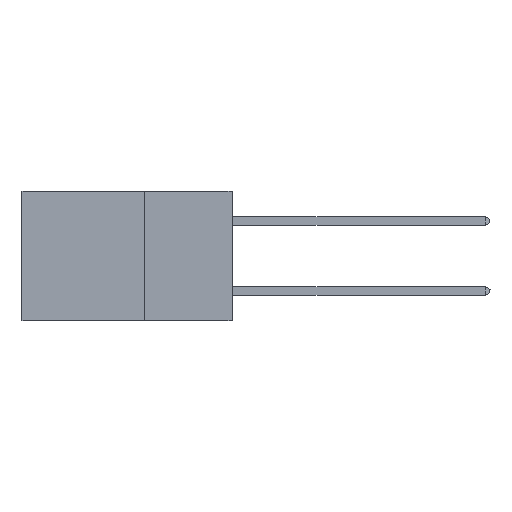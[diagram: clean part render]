
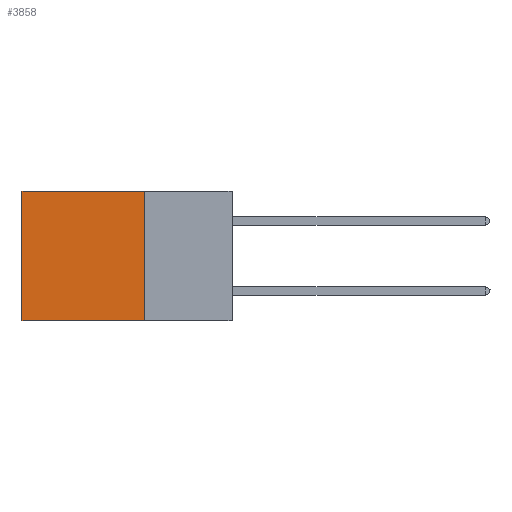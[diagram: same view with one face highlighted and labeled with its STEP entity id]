
A CAD part, left-side view. The second image highlights one B-rep face of the part: STEP entity #3858.
In plain terms, the highlighted planar face has unit normal (-1, 0, 0).
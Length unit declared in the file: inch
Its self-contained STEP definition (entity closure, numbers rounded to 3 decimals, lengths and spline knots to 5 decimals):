
#981 = ORIENTED_EDGE ( 'NONE', *, *, #20808, .T. ) ;
#1035 = DIRECTION ( 'NONE',  ( 0., 0., -1. ) ) ;
#1607 = ORIENTED_EDGE ( 'NONE', *, *, #6414, .T. ) ;
#1695 = DIRECTION ( 'NONE',  ( 0., 1., 0. ) ) ;
#2354 = VERTEX_POINT ( 'NONE', #20238 ) ;
#2769 = FACE_OUTER_BOUND ( 'NONE', #6070, .T. ) ;
#3026 = LINE ( 'NONE', #21168, #22658 ) ;
#3858 = ADVANCED_FACE ( 'NONE', ( #2769 ), #4705, .F. ) ;
#4690 = LINE ( 'NONE', #19210, #17046 ) ;
#4705 = PLANE ( 'NONE',  #22194 ) ;
#4819 = DIRECTION ( 'NONE',  ( 0., 1., 0. ) ) ;
#6070 = EDGE_LOOP ( 'NONE', ( #981, #16297, #16019, #1607 ) ) ;
#6388 = CARTESIAN_POINT ( 'NONE',  ( 0.2875, 0.25, -0.37 ) ) ;
#6414 = EDGE_CURVE ( 'NONE', #7320, #2354, #19826, .T. ) ;
#6417 = CARTESIAN_POINT ( 'NONE',  ( 0.2875, 0.25, 0. ) ) ;
#6467 = DIRECTION ( 'NONE',  ( 0., 0., -1. ) ) ;
#7256 = CARTESIAN_POINT ( 'NONE',  ( 0.2875, 0.25, 0. ) ) ;
#7320 = VERTEX_POINT ( 'NONE', #16934 ) ;
#9088 = VECTOR ( 'NONE', #4819, 39.37008 ) ;
#9526 = DIRECTION ( 'NONE',  ( 0., 0., -1. ) ) ;
#10051 = DIRECTION ( 'NONE',  ( 1., 0., 0. ) ) ;
#12334 = CARTESIAN_POINT ( 'NONE',  ( 0.2875, 0.6, -0.37 ) ) ;
#12747 = LINE ( 'NONE', #7256, #13029 ) ;
#13029 = VECTOR ( 'NONE', #9526, 39.37008 ) ;
#14997 = EDGE_CURVE ( 'NONE', #7320, #18546, #12747, .T. ) ;
#15842 = VERTEX_POINT ( 'NONE', #12334 ) ;
#16019 = ORIENTED_EDGE ( 'NONE', *, *, #14997, .F. ) ;
#16297 = ORIENTED_EDGE ( 'NONE', *, *, #23192, .F. ) ;
#16934 = CARTESIAN_POINT ( 'NONE',  ( 0.2875, 0.25, 0. ) ) ;
#17046 = VECTOR ( 'NONE', #6467, 39.37008 ) ;
#18546 = VERTEX_POINT ( 'NONE', #6388 ) ;
#19210 = CARTESIAN_POINT ( 'NONE',  ( 0.2875, 0.6, 0. ) ) ;
#19826 = LINE ( 'NONE', #22862, #9088 ) ;
#20238 = CARTESIAN_POINT ( 'NONE',  ( 0.2875, 0.6, 0. ) ) ;
#20808 = EDGE_CURVE ( 'NONE', #2354, #15842, #4690, .T. ) ;
#21168 = CARTESIAN_POINT ( 'NONE',  ( 0.2875, 0.25, -0.37 ) ) ;
#22194 = AXIS2_PLACEMENT_3D ( 'NONE', #6417, #10051, #1035 ) ;
#22658 = VECTOR ( 'NONE', #1695, 39.37008 ) ;
#22862 = CARTESIAN_POINT ( 'NONE',  ( 0.2875, 0.25, 0. ) ) ;
#23192 = EDGE_CURVE ( 'NONE', #18546, #15842, #3026, .T. ) ;
